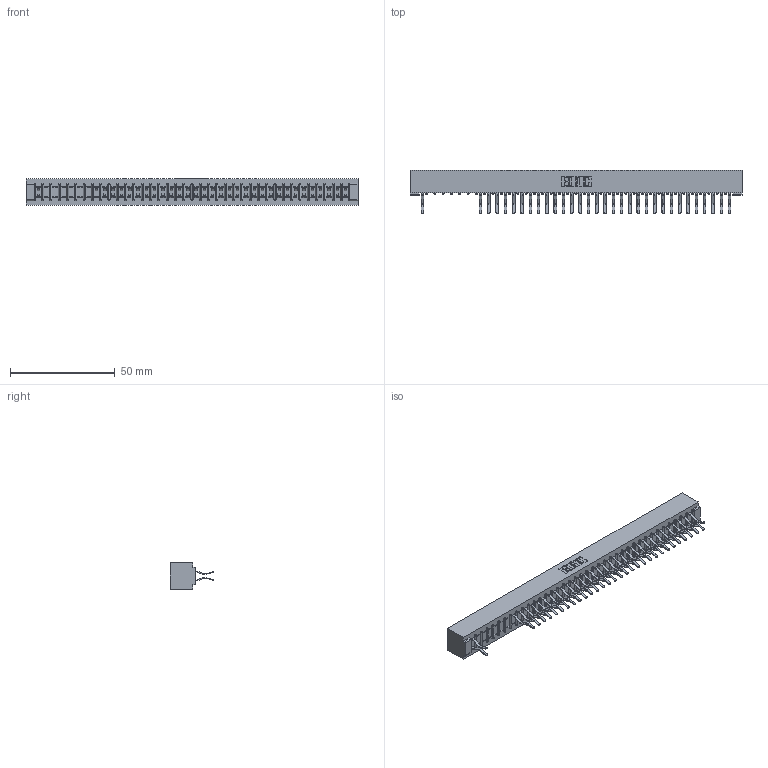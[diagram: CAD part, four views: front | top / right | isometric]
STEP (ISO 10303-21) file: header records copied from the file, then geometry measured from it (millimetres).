
FILE_DESCRIPTION (( 'STEP AP203' ), '1' );
FILE_NAME ('307-076-560-201.STEP', '2018-08-06T17:20:28', ( '' ), ( '' ), 'SwSTEP 2.0', 'SolidWorks 2016', '' );
FILE_SCHEMA (( 'CONFIG_CONTROL_DESIGN' ));
Length unit declared in the file: inch
Products named in the file (3): 307 Part_No Mounting Lugs; 307-290-001_560; 307-076-560-201
Assembly tree (64 placements, depth 2):
  307-076-560-201
    307 Part_No Mounting Lugs
    307-290-001_560  x63
Bounding box: 158.45 x 20.73 x 12.7 mm (x, y, z)
Volume: 17278.2 mm3; surface area: 20692.5 mm2
Topology: 64 solids, 64 shells, 3429 faces, 9661 edges, 6250 vertices
Faces by surface type: plane 2223, cylinder 1128, sphere 78
Entity records: 33696 total; most frequent: CARTESIAN_POINT 5565, ORIENTED_EDGE 5526, DIRECTION 5439, EDGE_CURVE 2763, VECTOR 2119, LINE 2119, VERTEX_POINT 1786, AXIS2_PLACEMENT_3D 1660
